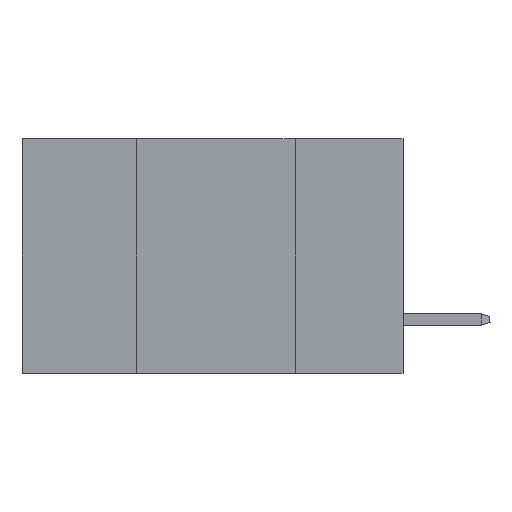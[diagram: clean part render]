
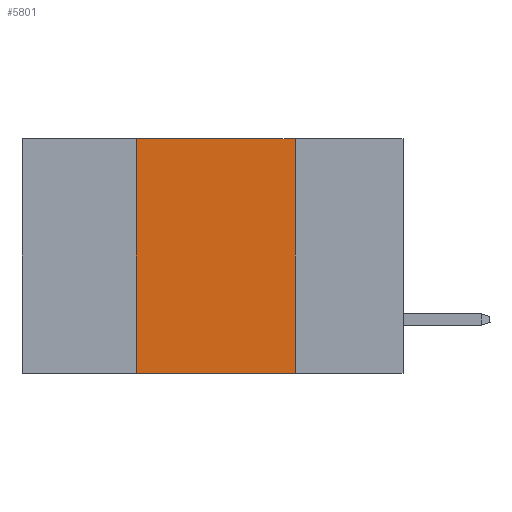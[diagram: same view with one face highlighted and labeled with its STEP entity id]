
A CAD part, left-side view. The second image highlights one B-rep face of the part: STEP entity #5801.
In plain terms, the highlighted planar face has unit normal (-1, 0, 0).
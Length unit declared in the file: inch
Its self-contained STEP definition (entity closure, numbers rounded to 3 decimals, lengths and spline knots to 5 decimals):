
#361 = CARTESIAN_POINT ( 'NONE',  ( 0., 0.6, 0. ) ) ;
#2494 = DIRECTION ( 'NONE',  ( 1., 0., 0. ) ) ;
#3119 = CARTESIAN_POINT ( 'NONE',  ( 0., 0.6, -0.37 ) ) ;
#3863 = DIRECTION ( 'NONE',  ( 0., -1., 0. ) ) ;
#3896 = EDGE_LOOP ( 'NONE', ( #9805, #12384, #14529, #22045 ) ) ;
#4033 = VECTOR ( 'NONE', #7004, 39.37008 ) ;
#4199 = CARTESIAN_POINT ( 'NONE',  ( 0., 0.17, 0. ) ) ;
#4468 = PLANE ( 'NONE',  #15260 ) ;
#5250 = CARTESIAN_POINT ( 'NONE',  ( 0., 0.17, -0.37 ) ) ;
#5801 = ADVANCED_FACE ( 'NONE', ( #15096 ), #4468, .F. ) ;
#6335 = LINE ( 'NONE', #20964, #17481 ) ;
#7004 = DIRECTION ( 'NONE',  ( 0., 0., -1. ) ) ;
#7111 = CARTESIAN_POINT ( 'NONE',  ( 0., 0.17, 0. ) ) ;
#8082 = DIRECTION ( 'NONE',  ( 0., 0., -1. ) ) ;
#8307 = CARTESIAN_POINT ( 'NONE',  ( 0., 0.6, 0. ) ) ;
#8644 = LINE ( 'NONE', #7111, #4033 ) ;
#9805 = ORIENTED_EDGE ( 'NONE', *, *, #19373, .F. ) ;
#10020 = LINE ( 'NONE', #3119, #11361 ) ;
#10288 = VECTOR ( 'NONE', #3863, 39.37008 ) ;
#11361 = VECTOR ( 'NONE', #17158, 39.37008 ) ;
#11681 = VERTEX_POINT ( 'NONE', #4199 ) ;
#12384 = ORIENTED_EDGE ( 'NONE', *, *, #15493, .F. ) ;
#13545 = CARTESIAN_POINT ( 'NONE',  ( 0., 0.42, 0. ) ) ;
#14053 = VERTEX_POINT ( 'NONE', #13545 ) ;
#14314 = EDGE_CURVE ( 'NONE', #22449, #16990, #10020, .T. ) ;
#14529 = ORIENTED_EDGE ( 'NONE', *, *, #17831, .F. ) ;
#15096 = FACE_OUTER_BOUND ( 'NONE', #3896, .T. ) ;
#15260 = AXIS2_PLACEMENT_3D ( 'NONE', #8307, #2494, #8082 ) ;
#15493 = EDGE_CURVE ( 'NONE', #14053, #11681, #16599, .T. ) ;
#15639 = CARTESIAN_POINT ( 'NONE',  ( 0., 0.42, -0.37 ) ) ;
#16599 = LINE ( 'NONE', #361, #10288 ) ;
#16990 = VERTEX_POINT ( 'NONE', #5250 ) ;
#17158 = DIRECTION ( 'NONE',  ( 0., -1., 0. ) ) ;
#17481 = VECTOR ( 'NONE', #19094, 39.37008 ) ;
#17831 = EDGE_CURVE ( 'NONE', #22449, #14053, #6335, .T. ) ;
#19094 = DIRECTION ( 'NONE',  ( 0., 0., 1. ) ) ;
#19373 = EDGE_CURVE ( 'NONE', #11681, #16990, #8644, .T. ) ;
#20964 = CARTESIAN_POINT ( 'NONE',  ( 0., 0.42, 0. ) ) ;
#22045 = ORIENTED_EDGE ( 'NONE', *, *, #14314, .T. ) ;
#22449 = VERTEX_POINT ( 'NONE', #15639 ) ;
